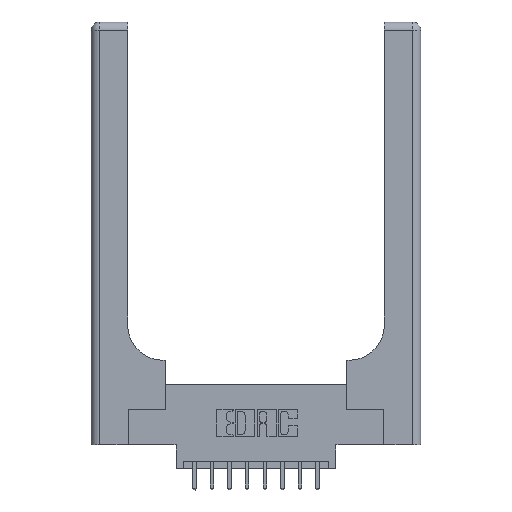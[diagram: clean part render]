
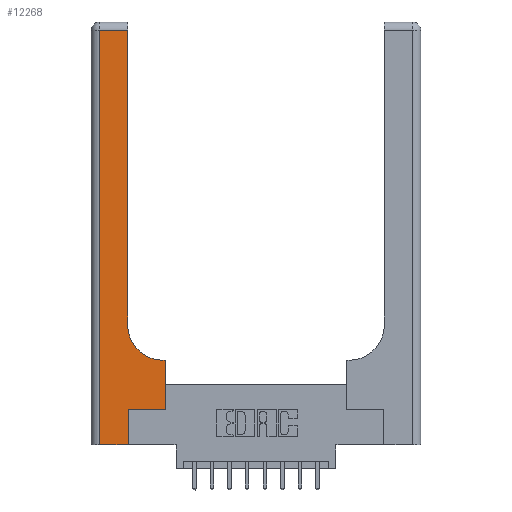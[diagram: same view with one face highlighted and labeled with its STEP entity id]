
A CAD part, top view. The second image highlights one B-rep face of the part: STEP entity #12268.
In plain terms, the highlighted planar face has unit normal (0, 0, 1).
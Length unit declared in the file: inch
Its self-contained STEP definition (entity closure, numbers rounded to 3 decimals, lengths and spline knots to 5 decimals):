
#308 = CARTESIAN_POINT ( 'NONE',  ( 0.265, 0., 0.37 ) ) ;
#492 = DIRECTION ( 'NONE',  ( 1., 0., 0. ) ) ;
#615 = EDGE_CURVE ( 'NONE', #10239, #5568, #3002, .T. ) ;
#648 = LINE ( 'NONE', #308, #9654 ) ;
#703 = PLANE ( 'NONE',  #6306 ) ;
#828 = ORIENTED_EDGE ( 'NONE', *, *, #1194, .T. ) ;
#873 = CARTESIAN_POINT ( 'NONE',  ( 0.51, 0.6, 0.37 ) ) ;
#1158 = VERTEX_POINT ( 'NONE', #4349 ) ;
#1194 = EDGE_CURVE ( 'NONE', #4152, #14090, #8697, .T. ) ;
#1571 = CARTESIAN_POINT ( 'NONE',  ( 0.265, 0.25, 0.37 ) ) ;
#1929 = EDGE_CURVE ( 'NONE', #5568, #13140, #2612, .T. ) ;
#1968 = ORIENTED_EDGE ( 'NONE', *, *, #7116, .T. ) ;
#2043 = CARTESIAN_POINT ( 'NONE',  ( 0.528, 0.25, 0.37 ) ) ;
#2123 = VECTOR ( 'NONE', #7471, 39.37008 ) ;
#2132 = EDGE_CURVE ( 'NONE', #3050, #1158, #6673, .T. ) ;
#2221 = CIRCLE ( 'NONE', #3587, 0.25 ) ;
#2612 = LINE ( 'NONE', #3628, #11959 ) ;
#2954 = EDGE_CURVE ( 'NONE', #7690, #3050, #2221, .T. ) ;
#3002 = LINE ( 'NONE', #4365, #3364 ) ;
#3050 = VERTEX_POINT ( 'NONE', #7026 ) ;
#3227 = DIRECTION ( 'NONE',  ( 0., 1., 0. ) ) ;
#3364 = VECTOR ( 'NONE', #12560, 39.37008 ) ;
#3587 = AXIS2_PLACEMENT_3D ( 'NONE', #12721, #5708, #13875 ) ;
#3628 = CARTESIAN_POINT ( 'NONE',  ( 0., 0., 0.37 ) ) ;
#3786 = ORIENTED_EDGE ( 'NONE', *, *, #2954, .T. ) ;
#3863 = VECTOR ( 'NONE', #492, 39.37008 ) ;
#3974 = VERTEX_POINT ( 'NONE', #1571 ) ;
#4107 = ORIENTED_EDGE ( 'NONE', *, *, #1929, .T. ) ;
#4152 = VERTEX_POINT ( 'NONE', #13540 ) ;
#4240 = LINE ( 'NONE', #14496, #3863 ) ;
#4249 = DIRECTION ( 'NONE',  ( -1., 0., 0. ) ) ;
#4349 = CARTESIAN_POINT ( 'NONE',  ( 0.26, 2.94, 0.37 ) ) ;
#4365 = CARTESIAN_POINT ( 'NONE',  ( 0.06, 3., 0.37 ) ) ;
#4774 = EDGE_CURVE ( 'NONE', #13140, #3974, #648, .T. ) ;
#5257 = ORIENTED_EDGE ( 'NONE', *, *, #2132, .T. ) ;
#5568 = VERTEX_POINT ( 'NONE', #13652 ) ;
#5708 = DIRECTION ( 'NONE',  ( 0., 0., -1. ) ) ;
#6121 = CARTESIAN_POINT ( 'NONE',  ( 0.265, 0., 0.37 ) ) ;
#6250 = ORIENTED_EDGE ( 'NONE', *, *, #4774, .T. ) ;
#6277 = CARTESIAN_POINT ( 'NONE',  ( 0.26, 0.6, 0.37 ) ) ;
#6306 = AXIS2_PLACEMENT_3D ( 'NONE', #10103, #11270, #4249 ) ;
#6673 = LINE ( 'NONE', #11050, #9036 ) ;
#7026 = CARTESIAN_POINT ( 'NONE',  ( 0.26, 0.85, 0.37 ) ) ;
#7116 = EDGE_CURVE ( 'NONE', #14090, #7690, #7658, .T. ) ;
#7384 = DIRECTION ( 'NONE',  ( 0., 1., 0. ) ) ;
#7440 = DIRECTION ( 'NONE',  ( -1., 0., 0. ) ) ;
#7471 = DIRECTION ( 'NONE',  ( -1., 0., 0. ) ) ;
#7658 = LINE ( 'NONE', #6277, #2123 ) ;
#7690 = VERTEX_POINT ( 'NONE', #873 ) ;
#7981 = VECTOR ( 'NONE', #3227, 39.37008 ) ;
#8156 = CARTESIAN_POINT ( 'NONE',  ( 0.528, 0.6, 0.37 ) ) ;
#8174 = CARTESIAN_POINT ( 'NONE',  ( 0.06, 2.94, 0.37 ) ) ;
#8324 = ORIENTED_EDGE ( 'NONE', *, *, #9880, .T. ) ;
#8697 = LINE ( 'NONE', #2043, #7981 ) ;
#9036 = VECTOR ( 'NONE', #12222, 39.37008 ) ;
#9585 = DIRECTION ( 'NONE',  ( 1., 0., 0. ) ) ;
#9654 = VECTOR ( 'NONE', #7384, 39.37008 ) ;
#9880 = EDGE_CURVE ( 'NONE', #3974, #4152, #4240, .T. ) ;
#9923 = ORIENTED_EDGE ( 'NONE', *, *, #14321, .T. ) ;
#10103 = CARTESIAN_POINT ( 'NONE',  ( 0., 3., 0.37 ) ) ;
#10239 = VERTEX_POINT ( 'NONE', #8174 ) ;
#10889 = CARTESIAN_POINT ( 'NONE',  ( 0., 2.94, 0.37 ) ) ;
#11050 = CARTESIAN_POINT ( 'NONE',  ( 0.26, 3., 0.37 ) ) ;
#11270 = DIRECTION ( 'NONE',  ( 0., 0., -1. ) ) ;
#11538 = FACE_OUTER_BOUND ( 'NONE', #13689, .T. ) ;
#11959 = VECTOR ( 'NONE', #9585, 39.37008 ) ;
#12222 = DIRECTION ( 'NONE',  ( 0., 1., 0. ) ) ;
#12268 = ADVANCED_FACE ( 'NONE', ( #11538 ), #703, .F. ) ;
#12560 = DIRECTION ( 'NONE',  ( 0., -1., 0. ) ) ;
#12721 = CARTESIAN_POINT ( 'NONE',  ( 0.51, 0.85, 0.37 ) ) ;
#13140 = VERTEX_POINT ( 'NONE', #6121 ) ;
#13540 = CARTESIAN_POINT ( 'NONE',  ( 0.528, 0.25, 0.37 ) ) ;
#13652 = CARTESIAN_POINT ( 'NONE',  ( 0.06, 0., 0.37 ) ) ;
#13689 = EDGE_LOOP ( 'NONE', ( #5257, #9923, #13708, #4107, #6250, #8324, #828, #1968, #3786 ) ) ;
#13708 = ORIENTED_EDGE ( 'NONE', *, *, #615, .T. ) ;
#13875 = DIRECTION ( 'NONE',  ( 1., 0., 0. ) ) ;
#13995 = VECTOR ( 'NONE', #7440, 39.37008 ) ;
#14090 = VERTEX_POINT ( 'NONE', #8156 ) ;
#14321 = EDGE_CURVE ( 'NONE', #1158, #10239, #14350, .T. ) ;
#14350 = LINE ( 'NONE', #10889, #13995 ) ;
#14496 = CARTESIAN_POINT ( 'NONE',  ( 0.265, 0.25, 0.37 ) ) ;
